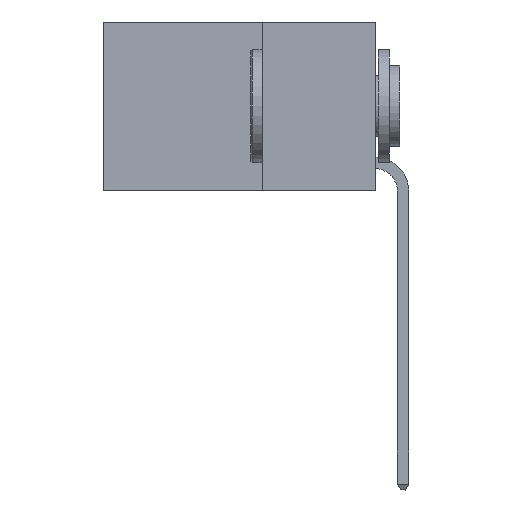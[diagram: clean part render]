
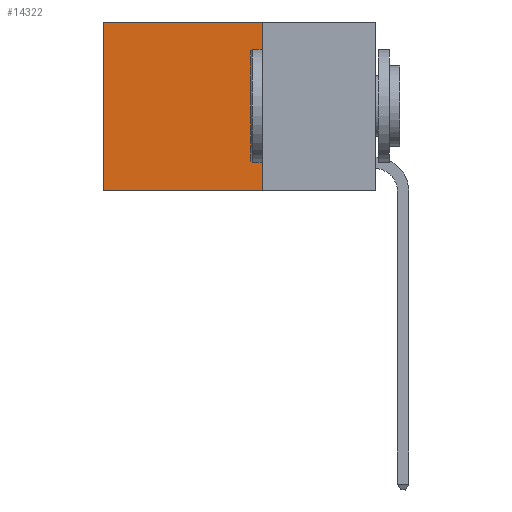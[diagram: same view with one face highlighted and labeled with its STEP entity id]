
A CAD part, left-side view. The second image highlights one B-rep face of the part: STEP entity #14322.
In plain terms, the highlighted planar face has unit normal (-1, 0, 0).
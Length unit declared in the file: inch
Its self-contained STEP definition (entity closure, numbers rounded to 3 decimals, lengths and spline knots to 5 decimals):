
#967 = CARTESIAN_POINT ( 'NONE',  ( 0.2625, 0.6, 0. ) ) ;
#1253 = CARTESIAN_POINT ( 'NONE',  ( 0.2625, 0.6, 0. ) ) ;
#1574 = VECTOR ( 'NONE', #5375, 39.37008 ) ;
#1702 = VERTEX_POINT ( 'NONE', #9491 ) ;
#1809 = CARTESIAN_POINT ( 'NONE',  ( 0.2625, 0.25, -0.37 ) ) ;
#2341 = LINE ( 'NONE', #11186, #9885 ) ;
#2715 = ORIENTED_EDGE ( 'NONE', *, *, #9569, .F. ) ;
#3658 = ORIENTED_EDGE ( 'NONE', *, *, #10023, .T. ) ;
#3702 = DIRECTION ( 'NONE',  ( 1., 0., 0. ) ) ;
#4751 = ORIENTED_EDGE ( 'NONE', *, *, #17093, .T. ) ;
#4977 = EDGE_CURVE ( 'NONE', #1702, #8414, #13930, .T. ) ;
#5375 = DIRECTION ( 'NONE',  ( 0., 0., -1. ) ) ;
#6097 = CARTESIAN_POINT ( 'NONE',  ( 0.2625, 0.6, -0.37 ) ) ;
#8414 = VERTEX_POINT ( 'NONE', #1809 ) ;
#9435 = VECTOR ( 'NONE', #13119, 39.37008 ) ;
#9491 = CARTESIAN_POINT ( 'NONE',  ( 0.2625, 0.25, 0. ) ) ;
#9569 = EDGE_CURVE ( 'NONE', #8414, #15199, #17522, .T. ) ;
#9885 = VECTOR ( 'NONE', #14114, 39.37008 ) ;
#10023 = EDGE_CURVE ( 'NONE', #1702, #13139, #2341, .T. ) ;
#10202 = CARTESIAN_POINT ( 'NONE',  ( 0.2625, 0.25, -0.37 ) ) ;
#10288 = DIRECTION ( 'NONE',  ( 0., 0., -1. ) ) ;
#10810 = EDGE_LOOP ( 'NONE', ( #4751, #2715, #13959, #3658 ) ) ;
#11164 = CARTESIAN_POINT ( 'NONE',  ( 0.2625, 0.25, 0. ) ) ;
#11186 = CARTESIAN_POINT ( 'NONE',  ( 0.2625, 0.25, 0. ) ) ;
#12753 = CARTESIAN_POINT ( 'NONE',  ( 0.2625, 0.25, 0. ) ) ;
#13119 = DIRECTION ( 'NONE',  ( 0., 1., 0. ) ) ;
#13139 = VERTEX_POINT ( 'NONE', #967 ) ;
#13930 = LINE ( 'NONE', #12753, #1574 ) ;
#13959 = ORIENTED_EDGE ( 'NONE', *, *, #4977, .F. ) ;
#14036 = PLANE ( 'NONE',  #15601 ) ;
#14092 = DIRECTION ( 'NONE',  ( 0., 0., -1. ) ) ;
#14114 = DIRECTION ( 'NONE',  ( 0., 1., 0. ) ) ;
#14322 = ADVANCED_FACE ( 'NONE', ( #16856 ), #14036, .F. ) ;
#15199 = VERTEX_POINT ( 'NONE', #6097 ) ;
#15601 = AXIS2_PLACEMENT_3D ( 'NONE', #11164, #3702, #14092 ) ;
#15676 = VECTOR ( 'NONE', #10288, 39.37008 ) ;
#16127 = LINE ( 'NONE', #1253, #15676 ) ;
#16856 = FACE_OUTER_BOUND ( 'NONE', #10810, .T. ) ;
#17093 = EDGE_CURVE ( 'NONE', #13139, #15199, #16127, .T. ) ;
#17522 = LINE ( 'NONE', #10202, #9435 ) ;
